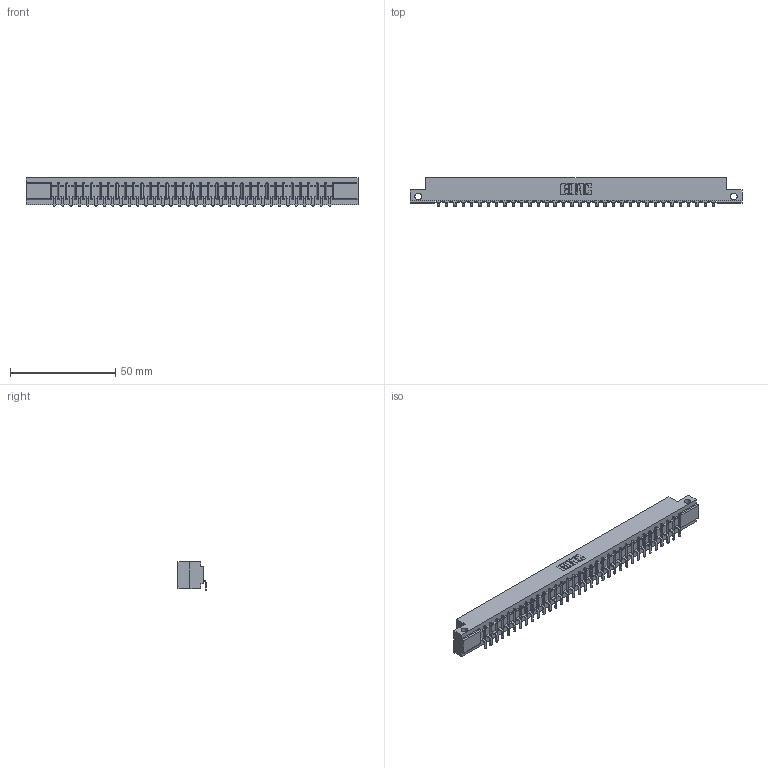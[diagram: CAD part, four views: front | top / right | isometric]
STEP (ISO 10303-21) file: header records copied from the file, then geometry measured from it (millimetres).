
FILE_DESCRIPTION (( 'STEP AP203' ), '1' );
FILE_NAME ('307-034-453-112.STEP', '2020-09-28T21:37:10', ( '' ), ( '' ), 'SwSTEP 2.0', 'SolidWorks 2020', '' );
FILE_SCHEMA (( 'CONFIG_CONTROL_DESIGN' ));
Length unit declared in the file: inch
Products named in the file (3): 307 Part_.128 Dia Side Mounting Holes; 307-034-453-112; 307-290-002_553
Assembly tree (35 placements, depth 2):
  307-034-453-112
    307 Part_.128 Dia Side Mounting Holes
    307-290-002_553  x34
Bounding box: 157.73 x 13.32 x 13.5 mm (x, y, z)
Volume: 16677.6 mm3; surface area: 20778 mm2
Topology: 35 solids, 35 shells, 2805 faces, 8619 edges, 5650 vertices
Faces by surface type: plane 1668, cylinder 1067, sphere 70
Entity records: 30990 total; most frequent: CARTESIAN_POINT 5228, ORIENTED_EDGE 5218, DIRECTION 5083, EDGE_CURVE 2609, VECTOR 1993, LINE 1993, VERTEX_POINT 1690, AXIS2_PLACEMENT_3D 1545
